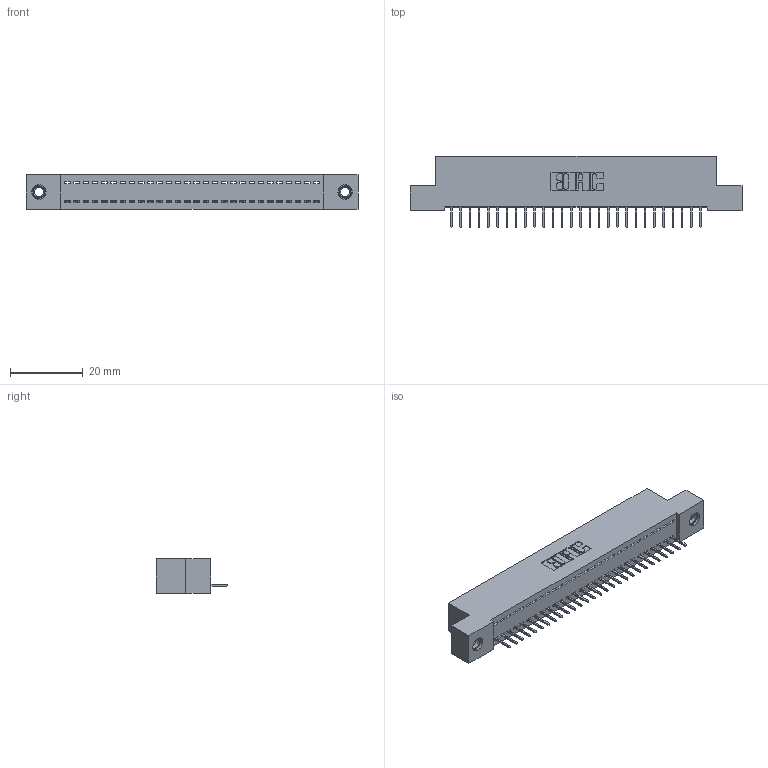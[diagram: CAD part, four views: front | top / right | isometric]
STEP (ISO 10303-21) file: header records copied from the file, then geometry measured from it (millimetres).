
FILE_DESCRIPTION (( 'STEP AP203' ), '1' );
FILE_NAME ('342-028-524-107.STEP', '2018-08-11T06:37:21', ( '' ), ( '' ), 'SwSTEP 2.0', 'SolidWorks 2016', '' );
FILE_SCHEMA (( 'CONFIG_CONTROL_DESIGN' ));
Length unit declared in the file: inch
Products named in the file (4): 345-292-001_345-293-124; 345-250-001_345-250-005-103; 342-028-524-107; 342 Part_TI
Assembly tree (31 placements, depth 2):
  342-028-524-107
    342 Part_TI
    345-292-001_345-293-124  x28
    345-250-001_345-250-005-103  x2
Bounding box: 91.44 x 19.69 x 9.4 mm (x, y, z)
Volume: 7842.6 mm3; surface area: 10943.7 mm2
Topology: 31 solids, 31 shells, 1906 faces, 5475 edges, 3530 vertices
Faces by surface type: plane 1442, cylinder 448, cone 12, torus 4
Entity records: 20056 total; most frequent: CARTESIAN_POINT 3441, ORIENTED_EDGE 3398, DIRECTION 2965, EDGE_CURVE 1699, LINE 1555, VECTOR 1555, VERTEX_POINT 1124, AXIS2_PLACEMENT_3D 705
